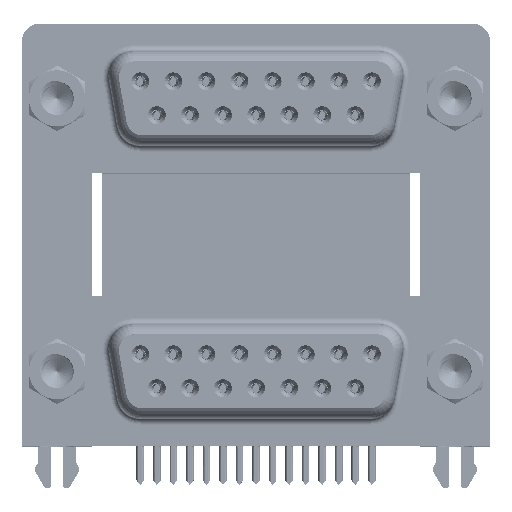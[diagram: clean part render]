
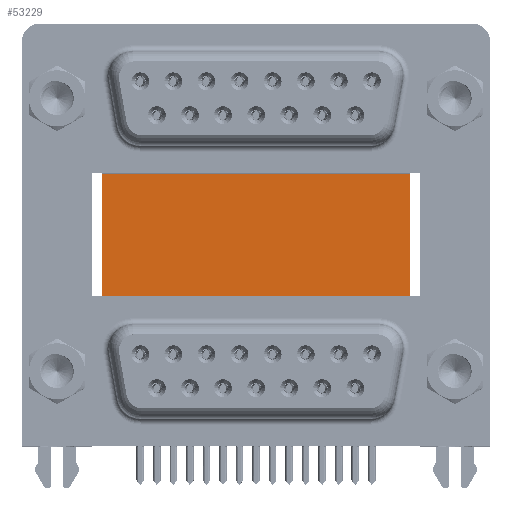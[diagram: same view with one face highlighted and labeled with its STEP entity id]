
A CAD part, top view. The second image highlights one B-rep face of the part: STEP entity #53229.
In plain terms, the highlighted planar face has unit normal (0, 0, 1).
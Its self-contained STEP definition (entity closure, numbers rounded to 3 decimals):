
#1008 = LINE ( 'NONE', #30513, #26003 ) ;
#3786 = LINE ( 'NONE', #38062, #13601 ) ;
#4186 = CARTESIAN_POINT ( 'NONE',  ( 29.58, -3.735, -12. ) ) ;
#5408 = AXIS2_PLACEMENT_3D ( 'NONE', #32456, #11375, #36374 ) ;
#7584 = CARTESIAN_POINT ( 'NONE',  ( 3.79, 16.585, -12. ) ) ;
#11375 = DIRECTION ( 'NONE',  ( 0., 0., -1. ) ) ;
#12502 = DIRECTION ( 'NONE',  ( 1., 0., 0. ) ) ;
#13601 = VECTOR ( 'NONE', #12502, 1000. ) ;
#13922 = EDGE_CURVE ( 'NONE', #27888, #27373, #13931, .T. ) ;
#13931 = LINE ( 'NONE', #31057, #39442 ) ;
#15581 = ORIENTED_EDGE ( 'NONE', *, *, #26296, .F. ) ;
#17057 = ORIENTED_EDGE ( 'NONE', *, *, #13922, .T. ) ;
#17966 = VERTEX_POINT ( 'NONE', #28611 ) ;
#22112 = VECTOR ( 'NONE', #50558, 1000. ) ;
#26003 = VECTOR ( 'NONE', #51292, 1000. ) ;
#26296 = EDGE_CURVE ( 'NONE', #17966, #27373, #1008, .T. ) ;
#27373 = VERTEX_POINT ( 'NONE', #4186 ) ;
#27888 = VERTEX_POINT ( 'NONE', #53488 ) ;
#28611 = CARTESIAN_POINT ( 'NONE',  ( 29.58, 16.585, -12. ) ) ;
#29533 = EDGE_LOOP ( 'NONE', ( #17057, #15581, #49303, #39901 ) ) ;
#30513 = CARTESIAN_POINT ( 'NONE',  ( 29.58, 16.585, -12. ) ) ;
#31057 = CARTESIAN_POINT ( 'NONE',  ( 3.79, -3.735, -12. ) ) ;
#32456 = CARTESIAN_POINT ( 'NONE',  ( 3.79, 16.585, -12. ) ) ;
#35528 = DIRECTION ( 'NONE',  ( 1., 0., 0. ) ) ;
#36374 = DIRECTION ( 'NONE',  ( -1., 0., 0. ) ) ;
#36914 = FACE_OUTER_BOUND ( 'NONE', #29533, .T. ) ;
#37604 = EDGE_CURVE ( 'NONE', #43339, #27888, #46063, .T. ) ;
#38062 = CARTESIAN_POINT ( 'NONE',  ( 3.79, 16.585, -12. ) ) ;
#39442 = VECTOR ( 'NONE', #35528, 1000. ) ;
#39901 = ORIENTED_EDGE ( 'NONE', *, *, #37604, .T. ) ;
#43339 = VERTEX_POINT ( 'NONE', #55438 ) ;
#46063 = LINE ( 'NONE', #7584, #22112 ) ;
#49040 = PLANE ( 'NONE',  #5408 ) ;
#49303 = ORIENTED_EDGE ( 'NONE', *, *, #54494, .F. ) ;
#50558 = DIRECTION ( 'NONE',  ( 0., -1., 0. ) ) ;
#51292 = DIRECTION ( 'NONE',  ( 0., -1., 0. ) ) ;
#53229 = ADVANCED_FACE ( 'NONE', ( #36914 ), #49040, .F. ) ;
#53488 = CARTESIAN_POINT ( 'NONE',  ( 3.79, -3.735, -12. ) ) ;
#54494 = EDGE_CURVE ( 'NONE', #43339, #17966, #3786, .T. ) ;
#55438 = CARTESIAN_POINT ( 'NONE',  ( 3.79, 16.585, -12. ) ) ;
